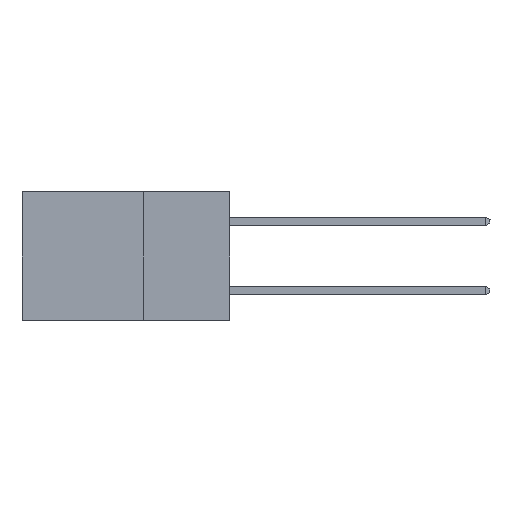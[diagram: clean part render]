
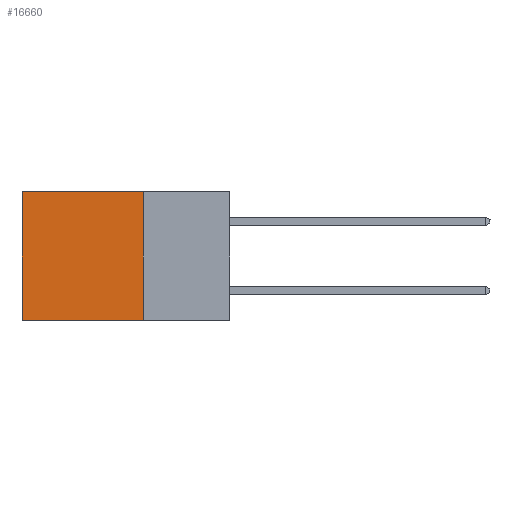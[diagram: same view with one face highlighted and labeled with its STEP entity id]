
A CAD part, left-side view. The second image highlights one B-rep face of the part: STEP entity #16660.
In plain terms, the highlighted planar face has unit normal (-1, 0, 0).
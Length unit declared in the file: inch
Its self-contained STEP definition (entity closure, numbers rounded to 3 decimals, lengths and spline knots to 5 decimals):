
#162 = DIRECTION ( 'NONE',  ( 0., 0., -1. ) ) ;
#383 = LINE ( 'NONE', #16333, #9076 ) ;
#467 = FACE_OUTER_BOUND ( 'NONE', #22560, .T. ) ;
#2102 = CARTESIAN_POINT ( 'NONE',  ( 0.2615, 0.25, -0.37 ) ) ;
#2575 = VECTOR ( 'NONE', #6418, 39.37008 ) ;
#3018 = DIRECTION ( 'NONE',  ( 1., 0., 0. ) ) ;
#3895 = ORIENTED_EDGE ( 'NONE', *, *, #20880, .T. ) ;
#4603 = LINE ( 'NONE', #6587, #11682 ) ;
#5291 = VERTEX_POINT ( 'NONE', #18199 ) ;
#6418 = DIRECTION ( 'NONE',  ( 0., 1., 0. ) ) ;
#6587 = CARTESIAN_POINT ( 'NONE',  ( 0.2615, 0.25, -0.37 ) ) ;
#7318 = CARTESIAN_POINT ( 'NONE',  ( 0.2615, 0.6, -0.37 ) ) ;
#8766 = AXIS2_PLACEMENT_3D ( 'NONE', #16636, #3018, #17191 ) ;
#8979 = CARTESIAN_POINT ( 'NONE',  ( 0.2615, 0.6, 0. ) ) ;
#9076 = VECTOR ( 'NONE', #162, 39.37008 ) ;
#9251 = LINE ( 'NONE', #2102, #18946 ) ;
#9532 = VERTEX_POINT ( 'NONE', #8979 ) ;
#9549 = ORIENTED_EDGE ( 'NONE', *, *, #15235, .F. ) ;
#9630 = ORIENTED_EDGE ( 'NONE', *, *, #10249, .T. ) ;
#10249 = EDGE_CURVE ( 'NONE', #11590, #9532, #22588, .T. ) ;
#10901 = VERTEX_POINT ( 'NONE', #7318 ) ;
#11590 = VERTEX_POINT ( 'NONE', #19445 ) ;
#11682 = VECTOR ( 'NONE', #20779, 39.37008 ) ;
#15235 = EDGE_CURVE ( 'NONE', #5291, #10901, #9251, .T. ) ;
#15441 = CARTESIAN_POINT ( 'NONE',  ( 0.2615, 0.25, 0. ) ) ;
#16333 = CARTESIAN_POINT ( 'NONE',  ( 0.2615, 0.6, -0.37 ) ) ;
#16636 = CARTESIAN_POINT ( 'NONE',  ( 0.2615, 0.25, -0.37 ) ) ;
#16660 = ADVANCED_FACE ( 'NONE', ( #467 ), #18400, .F. ) ;
#17191 = DIRECTION ( 'NONE',  ( 0., 0., -1. ) ) ;
#17201 = ORIENTED_EDGE ( 'NONE', *, *, #19628, .F. ) ;
#18199 = CARTESIAN_POINT ( 'NONE',  ( 0.2615, 0.25, -0.37 ) ) ;
#18400 = PLANE ( 'NONE',  #8766 ) ;
#18946 = VECTOR ( 'NONE', #22013, 39.37008 ) ;
#19445 = CARTESIAN_POINT ( 'NONE',  ( 0.2615, 0.25, 0. ) ) ;
#19628 = EDGE_CURVE ( 'NONE', #11590, #5291, #4603, .T. ) ;
#20779 = DIRECTION ( 'NONE',  ( 0., 0., -1. ) ) ;
#20880 = EDGE_CURVE ( 'NONE', #9532, #10901, #383, .T. ) ;
#22013 = DIRECTION ( 'NONE',  ( 0., 1., 0. ) ) ;
#22560 = EDGE_LOOP ( 'NONE', ( #3895, #9549, #17201, #9630 ) ) ;
#22588 = LINE ( 'NONE', #15441, #2575 ) ;
